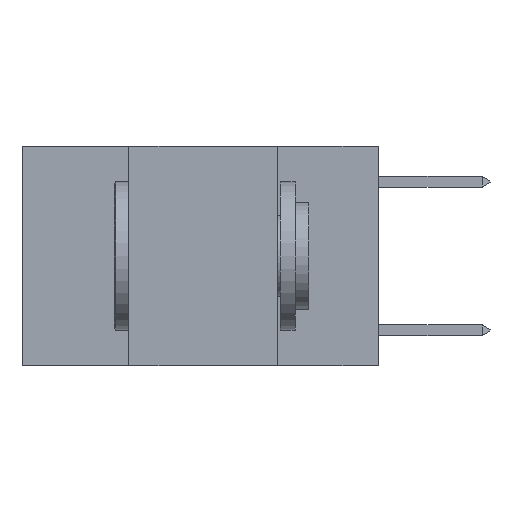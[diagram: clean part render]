
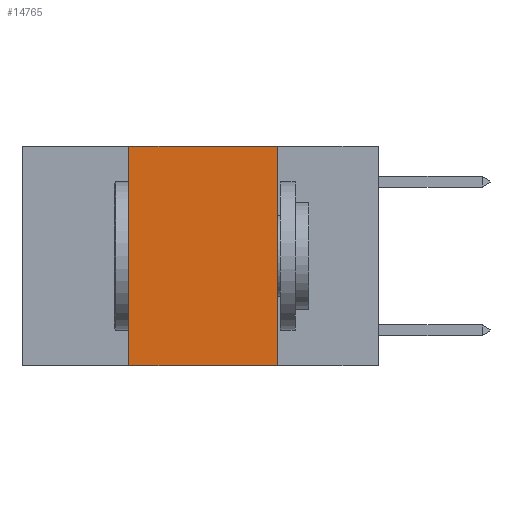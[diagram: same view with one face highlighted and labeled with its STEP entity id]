
A CAD part, left-side view. The second image highlights one B-rep face of the part: STEP entity #14765.
In plain terms, the highlighted planar face has unit normal (-1, 0, 0).
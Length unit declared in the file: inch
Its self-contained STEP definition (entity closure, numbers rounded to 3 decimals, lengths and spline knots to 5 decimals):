
#243 = EDGE_CURVE ( 'NONE', #3948, #14363, #13823, .T. ) ;
#608 = VECTOR ( 'NONE', #1064, 39.37008 ) ;
#1064 = DIRECTION ( 'NONE',  ( 0., -1., 0. ) ) ;
#1156 = ORIENTED_EDGE ( 'NONE', *, *, #6302, .T. ) ;
#1455 = VERTEX_POINT ( 'NONE', #7697 ) ;
#1734 = PLANE ( 'NONE',  #7434 ) ;
#1905 = VECTOR ( 'NONE', #9862, 39.37008 ) ;
#1972 = DIRECTION ( 'NONE',  ( 0., 0., 1. ) ) ;
#2034 = VERTEX_POINT ( 'NONE', #9231 ) ;
#2972 = EDGE_CURVE ( 'NONE', #1455, #3948, #4379, .T. ) ;
#3138 = CARTESIAN_POINT ( 'NONE',  ( 0., 0.6, 0. ) ) ;
#3149 = CARTESIAN_POINT ( 'NONE',  ( 0., 0.17, 0. ) ) ;
#3948 = VERTEX_POINT ( 'NONE', #5676 ) ;
#4223 = CARTESIAN_POINT ( 'NONE',  ( 0., 0.6, 0. ) ) ;
#4379 = LINE ( 'NONE', #10011, #4895 ) ;
#4471 = LINE ( 'NONE', #13836, #608 ) ;
#4895 = VECTOR ( 'NONE', #1972, 39.37008 ) ;
#5014 = LINE ( 'NONE', #6171, #1905 ) ;
#5676 = CARTESIAN_POINT ( 'NONE',  ( 0., 0.42, 0. ) ) ;
#6171 = CARTESIAN_POINT ( 'NONE',  ( 0., 0.17, 0. ) ) ;
#6302 = EDGE_CURVE ( 'NONE', #1455, #2034, #4471, .T. ) ;
#6312 = FACE_OUTER_BOUND ( 'NONE', #12515, .T. ) ;
#7203 = ORIENTED_EDGE ( 'NONE', *, *, #243, .F. ) ;
#7434 = AXIS2_PLACEMENT_3D ( 'NONE', #4223, #13666, #12188 ) ;
#7680 = ORIENTED_EDGE ( 'NONE', *, *, #2972, .F. ) ;
#7697 = CARTESIAN_POINT ( 'NONE',  ( 0., 0.42, -0.37 ) ) ;
#7857 = DIRECTION ( 'NONE',  ( 0., -1., 0. ) ) ;
#9231 = CARTESIAN_POINT ( 'NONE',  ( 0., 0.17, -0.37 ) ) ;
#9292 = VECTOR ( 'NONE', #7857, 39.37008 ) ;
#9346 = EDGE_CURVE ( 'NONE', #14363, #2034, #5014, .T. ) ;
#9862 = DIRECTION ( 'NONE',  ( 0., 0., -1. ) ) ;
#10011 = CARTESIAN_POINT ( 'NONE',  ( 0., 0.42, 0. ) ) ;
#12188 = DIRECTION ( 'NONE',  ( 0., 0., -1. ) ) ;
#12515 = EDGE_LOOP ( 'NONE', ( #13150, #7203, #7680, #1156 ) ) ;
#13150 = ORIENTED_EDGE ( 'NONE', *, *, #9346, .F. ) ;
#13666 = DIRECTION ( 'NONE',  ( 1., 0., 0. ) ) ;
#13823 = LINE ( 'NONE', #3138, #9292 ) ;
#13836 = CARTESIAN_POINT ( 'NONE',  ( 0., 0.6, -0.37 ) ) ;
#14363 = VERTEX_POINT ( 'NONE', #3149 ) ;
#14765 = ADVANCED_FACE ( 'NONE', ( #6312 ), #1734, .F. ) ;
